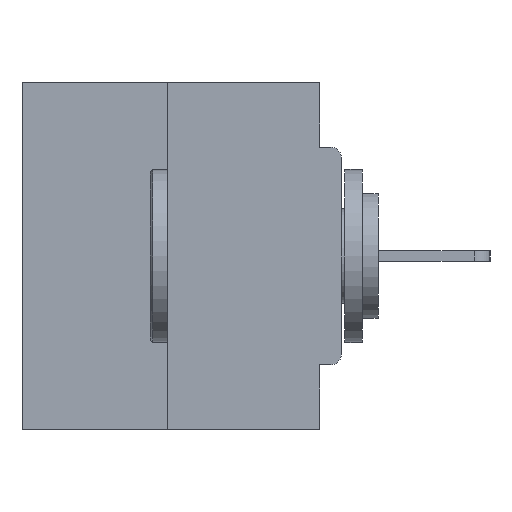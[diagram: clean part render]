
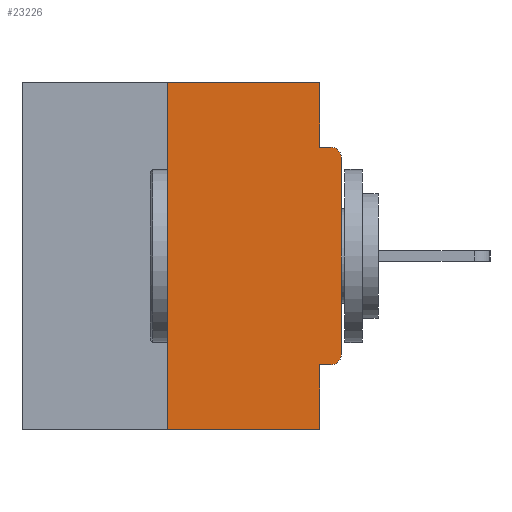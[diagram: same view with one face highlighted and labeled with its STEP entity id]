
A CAD part, left-side view. The second image highlights one B-rep face of the part: STEP entity #23226.
In plain terms, the highlighted planar face has unit normal (-1, 0, 0).
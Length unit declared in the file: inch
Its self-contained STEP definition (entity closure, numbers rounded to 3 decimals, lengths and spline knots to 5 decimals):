
#408 = DIRECTION ( 'NONE',  ( -1., 0., 0. ) ) ;
#853 = CARTESIAN_POINT ( 'NONE',  ( 0., 0., -0.1085 ) ) ;
#1564 = CARTESIAN_POINT ( 'NONE',  ( 0., 0.46, 0. ) ) ;
#2137 = AXIS2_PLACEMENT_3D ( 'NONE', #11534, #12015, #14145 ) ;
#2285 = LINE ( 'NONE', #9100, #12433 ) ;
#2746 = CARTESIAN_POINT ( 'NONE',  ( 0., 0., -0.3915 ) ) ;
#3063 = CIRCLE ( 'NONE', #19982, 0.015 ) ;
#3711 = DIRECTION ( 'NONE',  ( 0., -1., 0. ) ) ;
#4930 = EDGE_CURVE ( 'NONE', #20299, #24549, #28904, .T. ) ;
#5009 = VERTEX_POINT ( 'NONE', #16739 ) ;
#5084 = CARTESIAN_POINT ( 'NONE',  ( 0., 0.015, -0.3915 ) ) ;
#5177 = DIRECTION ( 'NONE',  ( 0., 0., -1. ) ) ;
#5328 = EDGE_CURVE ( 'NONE', #5009, #14010, #9678, .T. ) ;
#5594 = EDGE_CURVE ( 'NONE', #24549, #22728, #8256, .T. ) ;
#5669 = DIRECTION ( 'NONE',  ( -1., 0., 0. ) ) ;
#5781 = EDGE_CURVE ( 'NONE', #22669, #14010, #6544, .T. ) ;
#6544 = LINE ( 'NONE', #7606, #7526 ) ;
#7007 = ORIENTED_EDGE ( 'NONE', *, *, #12850, .F. ) ;
#7153 = EDGE_CURVE ( 'NONE', #22123, #22728, #3063, .T. ) ;
#7526 = VECTOR ( 'NONE', #5177, 39.37008 ) ;
#7606 = CARTESIAN_POINT ( 'NONE',  ( 0., 0.031, -0.5 ) ) ;
#7795 = CARTESIAN_POINT ( 'NONE',  ( 0., 0.015, -0.1085 ) ) ;
#7861 = CARTESIAN_POINT ( 'NONE',  ( 0., 0., -0.4065 ) ) ;
#8256 = LINE ( 'NONE', #26348, #8961 ) ;
#8409 = EDGE_CURVE ( 'NONE', #27206, #22123, #2285, .T. ) ;
#8961 = VECTOR ( 'NONE', #3711, 39.37008 ) ;
#9100 = CARTESIAN_POINT ( 'NONE',  ( 0., 0., 0. ) ) ;
#9203 = CARTESIAN_POINT ( 'NONE',  ( 0., 0.015, -0.0935 ) ) ;
#9255 = PLANE ( 'NONE',  #2137 ) ;
#9678 = LINE ( 'NONE', #18079, #27833 ) ;
#9690 = DIRECTION ( 'NONE',  ( 0., 0., 1. ) ) ;
#9809 = LINE ( 'NONE', #1564, #12980 ) ;
#11135 = CIRCLE ( 'NONE', #20501, 0.015 ) ;
#11477 = DIRECTION ( 'NONE',  ( 0., -1., 0. ) ) ;
#11534 = CARTESIAN_POINT ( 'NONE',  ( 0., 0.46, 0. ) ) ;
#11734 = DIRECTION ( 'NONE',  ( 0., 0., -1. ) ) ;
#11782 = VERTEX_POINT ( 'NONE', #19330 ) ;
#12015 = DIRECTION ( 'NONE',  ( 1., 0., 0. ) ) ;
#12311 = ORIENTED_EDGE ( 'NONE', *, *, #20024, .F. ) ;
#12433 = VECTOR ( 'NONE', #24518, 39.37008 ) ;
#12850 = EDGE_CURVE ( 'NONE', #25171, #20299, #9809, .T. ) ;
#12980 = VECTOR ( 'NONE', #23999, 39.37008 ) ;
#13350 = CARTESIAN_POINT ( 'NONE',  ( 0., 0.031, -0.4065 ) ) ;
#13914 = VECTOR ( 'NONE', #24665, 39.37008 ) ;
#14010 = VERTEX_POINT ( 'NONE', #26489 ) ;
#14145 = DIRECTION ( 'NONE',  ( 0., 0., -1. ) ) ;
#14480 = DIRECTION ( 'NONE',  ( 0., 1., 0. ) ) ;
#14757 = ORIENTED_EDGE ( 'NONE', *, *, #15119, .T. ) ;
#15119 = EDGE_CURVE ( 'NONE', #11782, #27206, #11135, .T. ) ;
#15695 = CARTESIAN_POINT ( 'NONE',  ( 0., 0.031, 0. ) ) ;
#16157 = ORIENTED_EDGE ( 'NONE', *, *, #16323, .F. ) ;
#16323 = EDGE_CURVE ( 'NONE', #11782, #22669, #18059, .T. ) ;
#16739 = CARTESIAN_POINT ( 'NONE',  ( 0., 0.25, -0.5 ) ) ;
#16952 = LINE ( 'NONE', #23057, #25061 ) ;
#18059 = LINE ( 'NONE', #7861, #27848 ) ;
#18076 = ORIENTED_EDGE ( 'NONE', *, *, #7153, .T. ) ;
#18079 = CARTESIAN_POINT ( 'NONE',  ( 0., 0.46, -0.5 ) ) ;
#19330 = CARTESIAN_POINT ( 'NONE',  ( 0., 0.015, -0.4065 ) ) ;
#19643 = ORIENTED_EDGE ( 'NONE', *, *, #5781, .F. ) ;
#19982 = AXIS2_PLACEMENT_3D ( 'NONE', #7795, #5669, #23391 ) ;
#20024 = EDGE_CURVE ( 'NONE', #5009, #25171, #16952, .T. ) ;
#20299 = VERTEX_POINT ( 'NONE', #26267 ) ;
#20501 = AXIS2_PLACEMENT_3D ( 'NONE', #5084, #408, #11734 ) ;
#22123 = VERTEX_POINT ( 'NONE', #853 ) ;
#22215 = EDGE_LOOP ( 'NONE', ( #7007, #12311, #27237, #19643, #16157, #14757, #27001, #18076, #22593, #27200 ) ) ;
#22593 = ORIENTED_EDGE ( 'NONE', *, *, #5594, .F. ) ;
#22669 = VERTEX_POINT ( 'NONE', #13350 ) ;
#22728 = VERTEX_POINT ( 'NONE', #9203 ) ;
#23057 = CARTESIAN_POINT ( 'NONE',  ( 0., 0.25, 0. ) ) ;
#23157 = CARTESIAN_POINT ( 'NONE',  ( 0., 0.031, -0.0935 ) ) ;
#23226 = ADVANCED_FACE ( 'NONE', ( #25739 ), #9255, .F. ) ;
#23391 = DIRECTION ( 'NONE',  ( 0., 0., -1. ) ) ;
#23999 = DIRECTION ( 'NONE',  ( 0., -1., 0. ) ) ;
#24518 = DIRECTION ( 'NONE',  ( 0., 0., 1. ) ) ;
#24549 = VERTEX_POINT ( 'NONE', #23157 ) ;
#24665 = DIRECTION ( 'NONE',  ( 0., 0., -1. ) ) ;
#25061 = VECTOR ( 'NONE', #9690, 39.37008 ) ;
#25171 = VERTEX_POINT ( 'NONE', #25891 ) ;
#25739 = FACE_OUTER_BOUND ( 'NONE', #22215, .T. ) ;
#25891 = CARTESIAN_POINT ( 'NONE',  ( 0., 0.25, 0. ) ) ;
#26267 = CARTESIAN_POINT ( 'NONE',  ( 0., 0.031, 0. ) ) ;
#26348 = CARTESIAN_POINT ( 'NONE',  ( 0., 0., -0.0935 ) ) ;
#26489 = CARTESIAN_POINT ( 'NONE',  ( 0., 0.031, -0.5 ) ) ;
#27001 = ORIENTED_EDGE ( 'NONE', *, *, #8409, .T. ) ;
#27200 = ORIENTED_EDGE ( 'NONE', *, *, #4930, .F. ) ;
#27206 = VERTEX_POINT ( 'NONE', #2746 ) ;
#27237 = ORIENTED_EDGE ( 'NONE', *, *, #5328, .T. ) ;
#27833 = VECTOR ( 'NONE', #11477, 39.37008 ) ;
#27848 = VECTOR ( 'NONE', #14480, 39.37008 ) ;
#28904 = LINE ( 'NONE', #15695, #13914 ) ;
